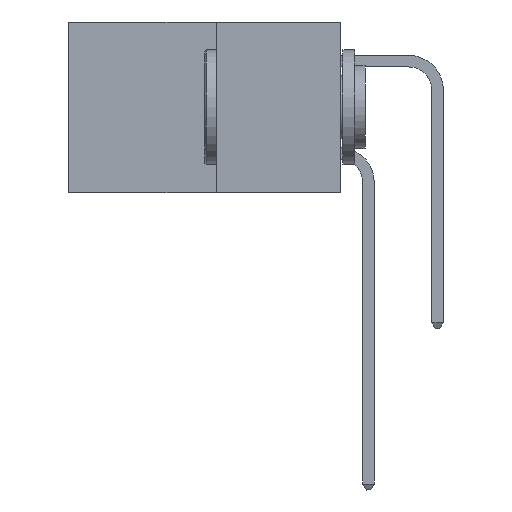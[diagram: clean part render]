
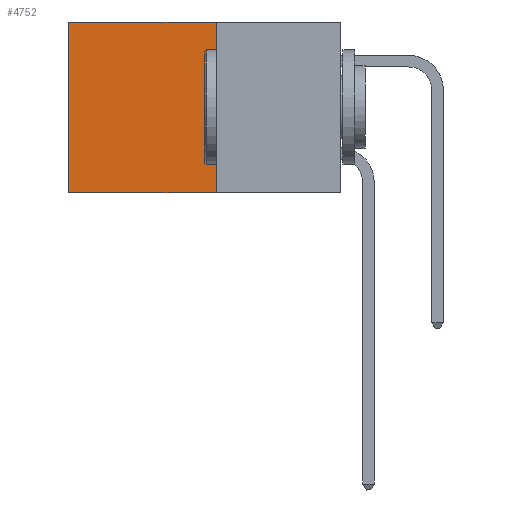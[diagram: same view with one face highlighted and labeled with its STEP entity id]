
A CAD part, left-side view. The second image highlights one B-rep face of the part: STEP entity #4752.
In plain terms, the highlighted planar face has unit normal (-1, 0, 0).
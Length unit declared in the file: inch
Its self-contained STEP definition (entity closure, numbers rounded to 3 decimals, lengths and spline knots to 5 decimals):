
#279 = CARTESIAN_POINT ( 'NONE',  ( 0.277, 0.27, -0.37 ) ) ;
#397 = DIRECTION ( 'NONE',  ( 0., 1., 0. ) ) ;
#449 = VERTEX_POINT ( 'NONE', #17353 ) ;
#1354 = DIRECTION ( 'NONE',  ( 1., 0., 0. ) ) ;
#1636 = VECTOR ( 'NONE', #6846, 39.37008 ) ;
#2150 = AXIS2_PLACEMENT_3D ( 'NONE', #23028, #1354, #22158 ) ;
#2239 = LINE ( 'NONE', #11981, #14342 ) ;
#2560 = VERTEX_POINT ( 'NONE', #25267 ) ;
#4042 = FACE_OUTER_BOUND ( 'NONE', #10217, .T. ) ;
#4752 = ADVANCED_FACE ( 'NONE', ( #4042 ), #24894, .F. ) ;
#5625 = CARTESIAN_POINT ( 'NONE',  ( 0.277, 0.59, -0.37 ) ) ;
#5639 = VECTOR ( 'NONE', #26757, 39.37008 ) ;
#6607 = LINE ( 'NONE', #11777, #5639 ) ;
#6846 = DIRECTION ( 'NONE',  ( 0., 0., -1. ) ) ;
#7869 = VERTEX_POINT ( 'NONE', #5625 ) ;
#8574 = ORIENTED_EDGE ( 'NONE', *, *, #12298, .F. ) ;
#10217 = EDGE_LOOP ( 'NONE', ( #21506, #12981, #8574, #14615 ) ) ;
#10442 = LINE ( 'NONE', #19643, #26843 ) ;
#10975 = EDGE_CURVE ( 'NONE', #449, #7869, #13861, .T. ) ;
#11777 = CARTESIAN_POINT ( 'NONE',  ( 0.277, 0.27, -0.37 ) ) ;
#11981 = CARTESIAN_POINT ( 'NONE',  ( 0.277, 0.27, -0.37 ) ) ;
#12298 = EDGE_CURVE ( 'NONE', #2560, #22585, #2239, .T. ) ;
#12981 = ORIENTED_EDGE ( 'NONE', *, *, #22835, .F. ) ;
#13861 = LINE ( 'NONE', #17405, #1636 ) ;
#14342 = VECTOR ( 'NONE', #24765, 39.37008 ) ;
#14615 = ORIENTED_EDGE ( 'NONE', *, *, #24804, .T. ) ;
#17353 = CARTESIAN_POINT ( 'NONE',  ( 0.277, 0.59, 0. ) ) ;
#17405 = CARTESIAN_POINT ( 'NONE',  ( 0.277, 0.59, -0.37 ) ) ;
#19643 = CARTESIAN_POINT ( 'NONE',  ( 0.277, 0.27, 0. ) ) ;
#21506 = ORIENTED_EDGE ( 'NONE', *, *, #10975, .T. ) ;
#22158 = DIRECTION ( 'NONE',  ( 0., 0., -1. ) ) ;
#22585 = VERTEX_POINT ( 'NONE', #279 ) ;
#22835 = EDGE_CURVE ( 'NONE', #22585, #7869, #6607, .T. ) ;
#23028 = CARTESIAN_POINT ( 'NONE',  ( 0.277, 0.27, -0.37 ) ) ;
#24765 = DIRECTION ( 'NONE',  ( 0., 0., -1. ) ) ;
#24804 = EDGE_CURVE ( 'NONE', #2560, #449, #10442, .T. ) ;
#24894 = PLANE ( 'NONE',  #2150 ) ;
#25267 = CARTESIAN_POINT ( 'NONE',  ( 0.277, 0.27, 0. ) ) ;
#26757 = DIRECTION ( 'NONE',  ( 0., 1., 0. ) ) ;
#26843 = VECTOR ( 'NONE', #397, 39.37008 ) ;
